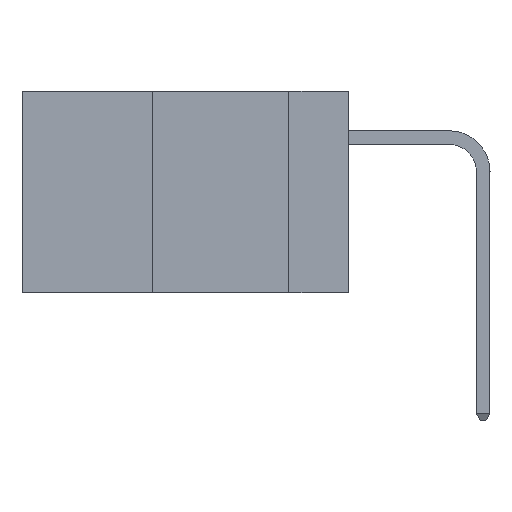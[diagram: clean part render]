
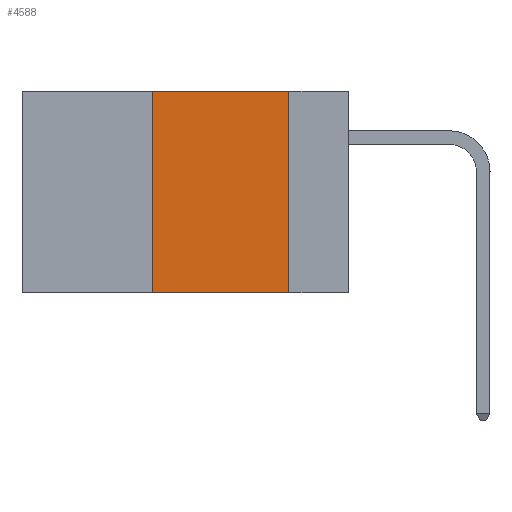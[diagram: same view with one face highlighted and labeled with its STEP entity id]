
A CAD part, left-side view. The second image highlights one B-rep face of the part: STEP entity #4588.
In plain terms, the highlighted planar face has unit normal (-1, 0, 0).
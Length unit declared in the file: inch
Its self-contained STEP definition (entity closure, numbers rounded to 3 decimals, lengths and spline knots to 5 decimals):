
#140 = ORIENTED_EDGE ( 'NONE', *, *, #3606, .F. ) ;
#277 = VECTOR ( 'NONE', #8117, 39.37008 ) ;
#1001 = CARTESIAN_POINT ( 'NONE',  ( 0., 0.6, -0.37 ) ) ;
#1961 = VERTEX_POINT ( 'NONE', #12352 ) ;
#1971 = CARTESIAN_POINT ( 'NONE',  ( 0., 0.6, 0. ) ) ;
#2144 = DIRECTION ( 'NONE',  ( 0., 0., -1. ) ) ;
#2146 = EDGE_LOOP ( 'NONE', ( #140, #8589, #11458, #11264 ) ) ;
#2299 = DIRECTION ( 'NONE',  ( 1., 0., 0. ) ) ;
#2588 = LINE ( 'NONE', #12128, #10052 ) ;
#2871 = EDGE_CURVE ( 'NONE', #11564, #7413, #8183, .T. ) ;
#2910 = VECTOR ( 'NONE', #6731, 39.37008 ) ;
#3606 = EDGE_CURVE ( 'NONE', #9459, #7413, #7691, .T. ) ;
#4309 = EDGE_CURVE ( 'NONE', #11564, #1961, #2588, .T. ) ;
#4588 = ADVANCED_FACE ( 'NONE', ( #7364 ), #6123, .F. ) ;
#5214 = VECTOR ( 'NONE', #9193, 39.37008 ) ;
#6123 = PLANE ( 'NONE',  #8772 ) ;
#6555 = DIRECTION ( 'NONE',  ( 0., 0., 1. ) ) ;
#6596 = CARTESIAN_POINT ( 'NONE',  ( 0., 0.11, 0. ) ) ;
#6731 = DIRECTION ( 'NONE',  ( 0., -1., 0. ) ) ;
#7364 = FACE_OUTER_BOUND ( 'NONE', #2146, .T. ) ;
#7413 = VERTEX_POINT ( 'NONE', #10871 ) ;
#7691 = LINE ( 'NONE', #9192, #5214 ) ;
#8117 = DIRECTION ( 'NONE',  ( 0., -1., 0. ) ) ;
#8183 = LINE ( 'NONE', #1001, #277 ) ;
#8589 = ORIENTED_EDGE ( 'NONE', *, *, #10781, .F. ) ;
#8772 = AXIS2_PLACEMENT_3D ( 'NONE', #1971, #2299, #2144 ) ;
#9192 = CARTESIAN_POINT ( 'NONE',  ( 0., 0.11, 0. ) ) ;
#9193 = DIRECTION ( 'NONE',  ( 0., 0., -1. ) ) ;
#9459 = VERTEX_POINT ( 'NONE', #6596 ) ;
#10052 = VECTOR ( 'NONE', #6555, 39.37008 ) ;
#10421 = CARTESIAN_POINT ( 'NONE',  ( 0., 0.36, -0.37 ) ) ;
#10781 = EDGE_CURVE ( 'NONE', #1961, #9459, #12593, .T. ) ;
#10871 = CARTESIAN_POINT ( 'NONE',  ( 0., 0.11, -0.37 ) ) ;
#11264 = ORIENTED_EDGE ( 'NONE', *, *, #2871, .T. ) ;
#11458 = ORIENTED_EDGE ( 'NONE', *, *, #4309, .F. ) ;
#11564 = VERTEX_POINT ( 'NONE', #10421 ) ;
#12128 = CARTESIAN_POINT ( 'NONE',  ( 0., 0.36, 0. ) ) ;
#12248 = CARTESIAN_POINT ( 'NONE',  ( 0., 0.6, 0. ) ) ;
#12352 = CARTESIAN_POINT ( 'NONE',  ( 0., 0.36, 0. ) ) ;
#12593 = LINE ( 'NONE', #12248, #2910 ) ;
